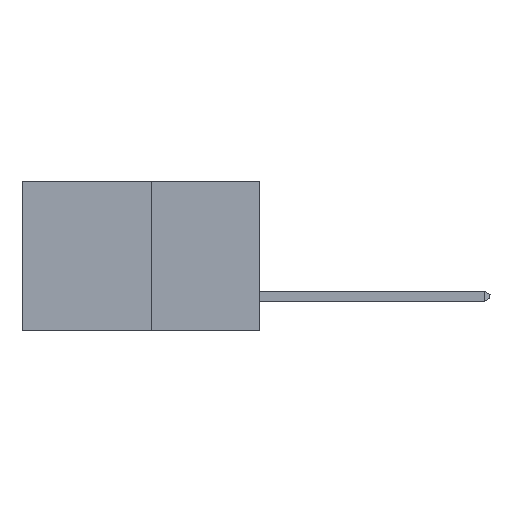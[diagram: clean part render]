
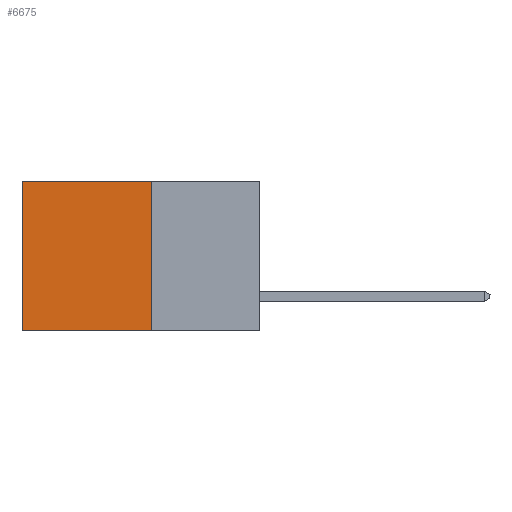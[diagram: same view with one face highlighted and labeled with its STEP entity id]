
A CAD part, left-side view. The second image highlights one B-rep face of the part: STEP entity #6675.
In plain terms, the highlighted planar face has unit normal (-1, 0, 0).
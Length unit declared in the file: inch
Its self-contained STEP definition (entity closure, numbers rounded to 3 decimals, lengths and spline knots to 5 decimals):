
#702 = VERTEX_POINT ( 'NONE', #15940 ) ;
#861 = LINE ( 'NONE', #7610, #14045 ) ;
#873 = DIRECTION ( 'NONE',  ( 0., 0., -1. ) ) ;
#947 = ORIENTED_EDGE ( 'NONE', *, *, #11618, .F. ) ;
#1048 = EDGE_LOOP ( 'NONE', ( #5374, #15882, #947, #2587 ) ) ;
#1357 = AXIS2_PLACEMENT_3D ( 'NONE', #7237, #6551, #6521 ) ;
#2075 = VECTOR ( 'NONE', #873, 39.37008 ) ;
#2234 = VERTEX_POINT ( 'NONE', #8618 ) ;
#2237 = VERTEX_POINT ( 'NONE', #9364 ) ;
#2587 = ORIENTED_EDGE ( 'NONE', *, *, #15130, .T. ) ;
#3460 = CARTESIAN_POINT ( 'NONE',  ( 0.277, 0.27, -0.37 ) ) ;
#4227 = EDGE_CURVE ( 'NONE', #702, #10259, #861, .T. ) ;
#5148 = VECTOR ( 'NONE', #14517, 39.37008 ) ;
#5374 = ORIENTED_EDGE ( 'NONE', *, *, #6415, .T. ) ;
#5496 = LINE ( 'NONE', #3460, #2075 ) ;
#5651 = CARTESIAN_POINT ( 'NONE',  ( 0.277, 0.27, 0. ) ) ;
#6415 = EDGE_CURVE ( 'NONE', #2237, #10259, #7339, .T. ) ;
#6521 = DIRECTION ( 'NONE',  ( 0., 0., -1. ) ) ;
#6551 = DIRECTION ( 'NONE',  ( 1., 0., 0. ) ) ;
#6645 = PLANE ( 'NONE',  #1357 ) ;
#6675 = ADVANCED_FACE ( 'NONE', ( #16442 ), #6645, .F. ) ;
#7237 = CARTESIAN_POINT ( 'NONE',  ( 0.277, 0.27, -0.37 ) ) ;
#7339 = LINE ( 'NONE', #9158, #13713 ) ;
#7551 = DIRECTION ( 'NONE',  ( 0., 1., 0. ) ) ;
#7610 = CARTESIAN_POINT ( 'NONE',  ( 0.277, 0.27, -0.37 ) ) ;
#8181 = CARTESIAN_POINT ( 'NONE',  ( 0.277, 0.59, -0.37 ) ) ;
#8618 = CARTESIAN_POINT ( 'NONE',  ( 0.277, 0.27, 0. ) ) ;
#9130 = DIRECTION ( 'NONE',  ( 0., 0., -1. ) ) ;
#9158 = CARTESIAN_POINT ( 'NONE',  ( 0.277, 0.59, -0.37 ) ) ;
#9364 = CARTESIAN_POINT ( 'NONE',  ( 0.277, 0.59, 0. ) ) ;
#10259 = VERTEX_POINT ( 'NONE', #8181 ) ;
#11618 = EDGE_CURVE ( 'NONE', #2234, #702, #5496, .T. ) ;
#13713 = VECTOR ( 'NONE', #9130, 39.37008 ) ;
#14045 = VECTOR ( 'NONE', #7551, 39.37008 ) ;
#14517 = DIRECTION ( 'NONE',  ( 0., 1., 0. ) ) ;
#14869 = LINE ( 'NONE', #5651, #5148 ) ;
#15130 = EDGE_CURVE ( 'NONE', #2234, #2237, #14869, .T. ) ;
#15882 = ORIENTED_EDGE ( 'NONE', *, *, #4227, .F. ) ;
#15940 = CARTESIAN_POINT ( 'NONE',  ( 0.277, 0.27, -0.37 ) ) ;
#16442 = FACE_OUTER_BOUND ( 'NONE', #1048, .T. ) ;
